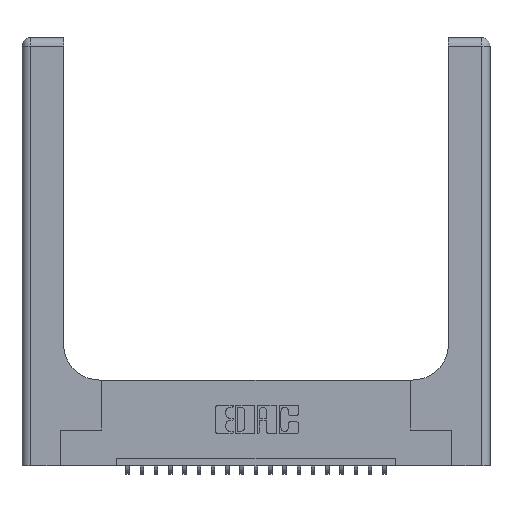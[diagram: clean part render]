
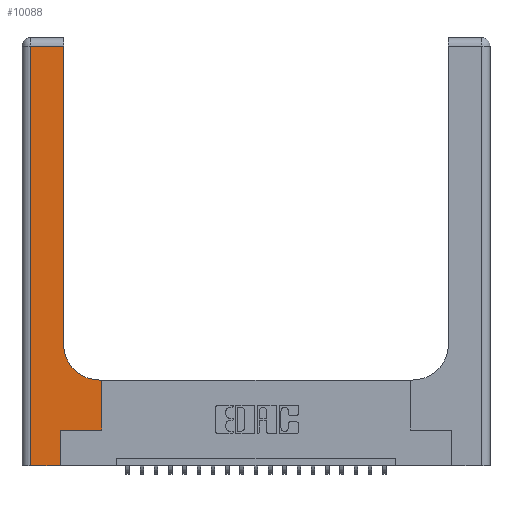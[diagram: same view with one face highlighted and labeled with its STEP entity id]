
A CAD part, top view. The second image highlights one B-rep face of the part: STEP entity #10088.
In plain terms, the highlighted planar face has unit normal (0, 0, 1).
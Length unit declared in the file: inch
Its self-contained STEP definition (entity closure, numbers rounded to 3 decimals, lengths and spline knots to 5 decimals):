
#19 = VERTEX_POINT ( 'NONE', #11382 ) ;
#181 = EDGE_CURVE ( 'NONE', #4219, #19592, #8892, .T. ) ;
#1063 = VECTOR ( 'NONE', #11725, 39.37008 ) ;
#1346 = AXIS2_PLACEMENT_3D ( 'NONE', #17645, #22537, #1963 ) ;
#1963 = DIRECTION ( 'NONE',  ( -1., 0., 0. ) ) ;
#2271 = EDGE_CURVE ( 'NONE', #20823, #15361, #9254, .T. ) ;
#2630 = VECTOR ( 'NONE', #18847, 39.37008 ) ;
#3310 = CARTESIAN_POINT ( 'NONE',  ( 0.5415, 0.6, 0.37 ) ) ;
#3639 = CARTESIAN_POINT ( 'NONE',  ( 0.2915, 3., 0.37 ) ) ;
#3930 = VECTOR ( 'NONE', #7736, 39.37008 ) ;
#4219 = VERTEX_POINT ( 'NONE', #16697 ) ;
#4267 = VECTOR ( 'NONE', #22687, 39.37008 ) ;
#4759 = DIRECTION ( 'NONE',  ( -1., 0., 0. ) ) ;
#4880 = DIRECTION ( 'NONE',  ( 1., 0., 0. ) ) ;
#4916 = CARTESIAN_POINT ( 'NONE',  ( 0.2915, 2.94, 0.37 ) ) ;
#5544 = ORIENTED_EDGE ( 'NONE', *, *, #7858, .T. ) ;
#5725 = CARTESIAN_POINT ( 'NONE',  ( 0.5585, 0.25, 0.37 ) ) ;
#5976 = CARTESIAN_POINT ( 'NONE',  ( 0.06, 3., 0.37 ) ) ;
#6240 = VECTOR ( 'NONE', #4880, 39.37008 ) ;
#6489 = VERTEX_POINT ( 'NONE', #20133 ) ;
#7016 = EDGE_CURVE ( 'NONE', #19592, #19064, #21581, .T. ) ;
#7123 = DIRECTION ( 'NONE',  ( 0., 1., 0. ) ) ;
#7393 = LINE ( 'NONE', #22122, #1063 ) ;
#7413 = CARTESIAN_POINT ( 'NONE',  ( 0., 0., 0.37 ) ) ;
#7736 = DIRECTION ( 'NONE',  ( 0., -1., 0. ) ) ;
#7858 = EDGE_CURVE ( 'NONE', #19064, #13968, #20438, .T. ) ;
#7899 = CARTESIAN_POINT ( 'NONE',  ( 0.2915, 0.85, 0.37 ) ) ;
#7973 = PLANE ( 'NONE',  #1346 ) ;
#8206 = ORIENTED_EDGE ( 'NONE', *, *, #13939, .T. ) ;
#8346 = VECTOR ( 'NONE', #21539, 39.37008 ) ;
#8892 = LINE ( 'NONE', #7413, #8346 ) ;
#9254 = LINE ( 'NONE', #3639, #4267 ) ;
#9327 = EDGE_CURVE ( 'NONE', #13968, #19, #7393, .T. ) ;
#9433 = CARTESIAN_POINT ( 'NONE',  ( 0.269, 0., 0.37 ) ) ;
#10088 = ADVANCED_FACE ( 'NONE', ( #15053 ), #7973, .F. ) ;
#10117 = CARTESIAN_POINT ( 'NONE',  ( 0.5415, 0.85, 0.37 ) ) ;
#10739 = ORIENTED_EDGE ( 'NONE', *, *, #12746, .T. ) ;
#11276 = EDGE_CURVE ( 'NONE', #19, #14663, #21236, .T. ) ;
#11382 = CARTESIAN_POINT ( 'NONE',  ( 0.5585, 0.6, 0.37 ) ) ;
#11653 = CARTESIAN_POINT ( 'NONE',  ( 0., 2.94, 0.37 ) ) ;
#11725 = DIRECTION ( 'NONE',  ( 0., 1., 0. ) ) ;
#11786 = ORIENTED_EDGE ( 'NONE', *, *, #11276, .T. ) ;
#11938 = ORIENTED_EDGE ( 'NONE', *, *, #9327, .T. ) ;
#12317 = CARTESIAN_POINT ( 'NONE',  ( 0.269, 0., 0.37 ) ) ;
#12672 = ORIENTED_EDGE ( 'NONE', *, *, #181, .T. ) ;
#12746 = EDGE_CURVE ( 'NONE', #14663, #20823, #14683, .T. ) ;
#13190 = AXIS2_PLACEMENT_3D ( 'NONE', #10117, #13543, #22364 ) ;
#13543 = DIRECTION ( 'NONE',  ( 0., 0., -1. ) ) ;
#13545 = CARTESIAN_POINT ( 'NONE',  ( 0.269, 0.25, 0.37 ) ) ;
#13802 = EDGE_LOOP ( 'NONE', ( #18827, #18289, #8206, #12672, #18213, #5544, #11938, #11786, #10739 ) ) ;
#13939 = EDGE_CURVE ( 'NONE', #6489, #4219, #17855, .T. ) ;
#13968 = VERTEX_POINT ( 'NONE', #5725 ) ;
#14210 = LINE ( 'NONE', #11653, #18015 ) ;
#14663 = VERTEX_POINT ( 'NONE', #3310 ) ;
#14683 = CIRCLE ( 'NONE', #13190, 0.25 ) ;
#15053 = FACE_OUTER_BOUND ( 'NONE', #13802, .T. ) ;
#15361 = VERTEX_POINT ( 'NONE', #4916 ) ;
#16697 = CARTESIAN_POINT ( 'NONE',  ( 0.06, 0., 0.37 ) ) ;
#17645 = CARTESIAN_POINT ( 'NONE',  ( 0., 3., 0.37 ) ) ;
#17855 = LINE ( 'NONE', #5976, #3930 ) ;
#18015 = VECTOR ( 'NONE', #4759, 39.37008 ) ;
#18213 = ORIENTED_EDGE ( 'NONE', *, *, #7016, .T. ) ;
#18289 = ORIENTED_EDGE ( 'NONE', *, *, #19534, .T. ) ;
#18827 = ORIENTED_EDGE ( 'NONE', *, *, #2271, .T. ) ;
#18847 = DIRECTION ( 'NONE',  ( -1., 0., 0. ) ) ;
#19064 = VERTEX_POINT ( 'NONE', #13545 ) ;
#19534 = EDGE_CURVE ( 'NONE', #15361, #6489, #14210, .T. ) ;
#19592 = VERTEX_POINT ( 'NONE', #9433 ) ;
#20133 = CARTESIAN_POINT ( 'NONE',  ( 0.06, 2.94, 0.37 ) ) ;
#20438 = LINE ( 'NONE', #20696, #6240 ) ;
#20696 = CARTESIAN_POINT ( 'NONE',  ( 0.269, 0.25, 0.37 ) ) ;
#20823 = VERTEX_POINT ( 'NONE', #7899 ) ;
#21029 = VECTOR ( 'NONE', #7123, 39.37008 ) ;
#21236 = LINE ( 'NONE', #22369, #2630 ) ;
#21539 = DIRECTION ( 'NONE',  ( 1., 0., 0. ) ) ;
#21581 = LINE ( 'NONE', #12317, #21029 ) ;
#22122 = CARTESIAN_POINT ( 'NONE',  ( 0.5585, 0.25, 0.37 ) ) ;
#22364 = DIRECTION ( 'NONE',  ( 1., 0., 0. ) ) ;
#22369 = CARTESIAN_POINT ( 'NONE',  ( 0.2915, 0.6, 0.37 ) ) ;
#22537 = DIRECTION ( 'NONE',  ( 0., 0., -1. ) ) ;
#22687 = DIRECTION ( 'NONE',  ( 0., 1., 0. ) ) ;
